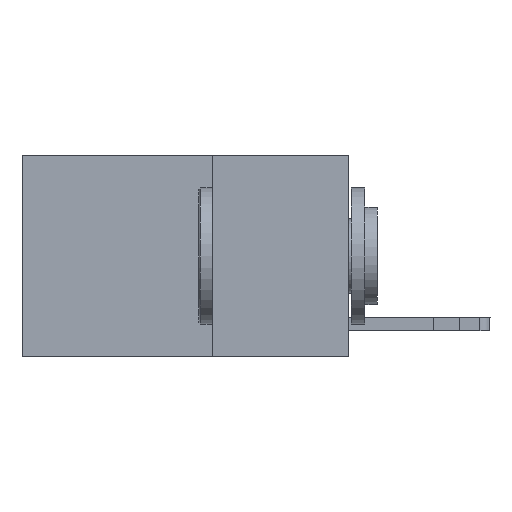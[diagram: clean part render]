
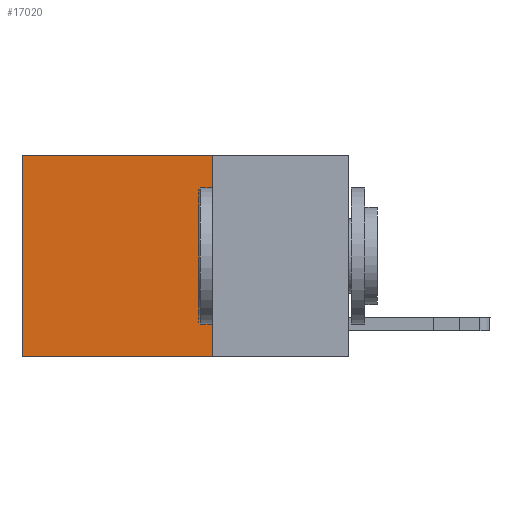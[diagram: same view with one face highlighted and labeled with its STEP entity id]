
A CAD part, left-side view. The second image highlights one B-rep face of the part: STEP entity #17020.
In plain terms, the highlighted planar face has unit normal (-1, 0, 0).
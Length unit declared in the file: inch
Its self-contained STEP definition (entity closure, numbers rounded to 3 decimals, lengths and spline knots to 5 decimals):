
#51 = EDGE_CURVE ( 'NONE', #2591, #20269, #13383, .T. ) ;
#186 = CARTESIAN_POINT ( 'NONE',  ( 0.2625, 0.25, -0.37 ) ) ;
#687 = PLANE ( 'NONE',  #10589 ) ;
#2591 = VERTEX_POINT ( 'NONE', #7447 ) ;
#2690 = DIRECTION ( 'NONE',  ( 0., 0., -1. ) ) ;
#3227 = CARTESIAN_POINT ( 'NONE',  ( 0.2625, 0.25, -0.37 ) ) ;
#3639 = LINE ( 'NONE', #21308, #17512 ) ;
#4454 = VERTEX_POINT ( 'NONE', #3227 ) ;
#4894 = EDGE_CURVE ( 'NONE', #18648, #4454, #19022, .T. ) ;
#6133 = CARTESIAN_POINT ( 'NONE',  ( 0.2625, 0.25, 0. ) ) ;
#6196 = ORIENTED_EDGE ( 'NONE', *, *, #10883, .T. ) ;
#6402 = DIRECTION ( 'NONE',  ( 0., 1., 0. ) ) ;
#7447 = CARTESIAN_POINT ( 'NONE',  ( 0.2625, 0.6, 0. ) ) ;
#7692 = CARTESIAN_POINT ( 'NONE',  ( 0.2625, 0.25, 0. ) ) ;
#9008 = VECTOR ( 'NONE', #11776, 39.37008 ) ;
#9679 = EDGE_CURVE ( 'NONE', #4454, #20269, #18175, .T. ) ;
#10589 = AXIS2_PLACEMENT_3D ( 'NONE', #12095, #14026, #2690 ) ;
#10883 = EDGE_CURVE ( 'NONE', #18648, #2591, #3639, .T. ) ;
#11776 = DIRECTION ( 'NONE',  ( 0., 0., -1. ) ) ;
#12095 = CARTESIAN_POINT ( 'NONE',  ( 0.2625, 0.25, 0. ) ) ;
#12676 = ORIENTED_EDGE ( 'NONE', *, *, #9679, .F. ) ;
#13187 = VECTOR ( 'NONE', #19048, 39.37008 ) ;
#13383 = LINE ( 'NONE', #14621, #18360 ) ;
#14026 = DIRECTION ( 'NONE',  ( 1., 0., 0. ) ) ;
#14483 = DIRECTION ( 'NONE',  ( 0., 0., -1. ) ) ;
#14621 = CARTESIAN_POINT ( 'NONE',  ( 0.2625, 0.6, 0. ) ) ;
#17020 = ADVANCED_FACE ( 'NONE', ( #19234 ), #687, .F. ) ;
#17512 = VECTOR ( 'NONE', #6402, 39.37008 ) ;
#18175 = LINE ( 'NONE', #186, #13187 ) ;
#18360 = VECTOR ( 'NONE', #14483, 39.37008 ) ;
#18648 = VERTEX_POINT ( 'NONE', #7692 ) ;
#19022 = LINE ( 'NONE', #6133, #9008 ) ;
#19048 = DIRECTION ( 'NONE',  ( 0., 1., 0. ) ) ;
#19234 = FACE_OUTER_BOUND ( 'NONE', #24142, .T. ) ;
#20022 = CARTESIAN_POINT ( 'NONE',  ( 0.2625, 0.6, -0.37 ) ) ;
#20269 = VERTEX_POINT ( 'NONE', #20022 ) ;
#21308 = CARTESIAN_POINT ( 'NONE',  ( 0.2625, 0.25, 0. ) ) ;
#23009 = ORIENTED_EDGE ( 'NONE', *, *, #51, .T. ) ;
#23040 = ORIENTED_EDGE ( 'NONE', *, *, #4894, .F. ) ;
#24142 = EDGE_LOOP ( 'NONE', ( #23009, #12676, #23040, #6196 ) ) ;
